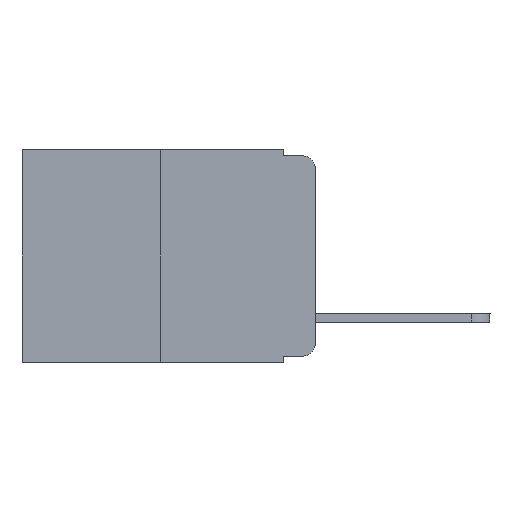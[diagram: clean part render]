
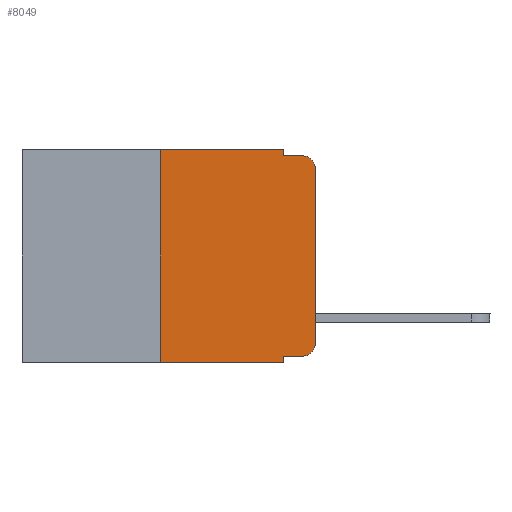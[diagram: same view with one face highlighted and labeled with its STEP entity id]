
A CAD part, left-side view. The second image highlights one B-rep face of the part: STEP entity #8049.
In plain terms, the highlighted planar face has unit normal (-1, 0, 0).
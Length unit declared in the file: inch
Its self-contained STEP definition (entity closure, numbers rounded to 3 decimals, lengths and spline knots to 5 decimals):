
#167 = VECTOR ( 'NONE', #13975, 39.37008 ) ;
#238 = EDGE_CURVE ( 'NONE', #725, #4307, #11123, .T. ) ;
#259 = LINE ( 'NONE', #12932, #1008 ) ;
#273 = LINE ( 'NONE', #460, #11075 ) ;
#423 = VERTEX_POINT ( 'NONE', #4367 ) ;
#460 = CARTESIAN_POINT ( 'NONE',  ( 0., 0.473, 0. ) ) ;
#542 = LINE ( 'NONE', #11695, #167 ) ;
#674 = EDGE_CURVE ( 'NONE', #6164, #3727, #14731, .T. ) ;
#712 = CARTESIAN_POINT ( 'NONE',  ( 0., 0.02, -0.01 ) ) ;
#725 = VERTEX_POINT ( 'NONE', #7876 ) ;
#894 = ORIENTED_EDGE ( 'NONE', *, *, #15032, .T. ) ;
#1008 = VECTOR ( 'NONE', #12884, 39.37008 ) ;
#1167 = DIRECTION ( 'NONE',  ( 0., 0., -1. ) ) ;
#1240 = VECTOR ( 'NONE', #3168, 39.37008 ) ;
#1358 = CARTESIAN_POINT ( 'NONE',  ( 0., 0.473, -0.343 ) ) ;
#1470 = CARTESIAN_POINT ( 'NONE',  ( 0., 0.051, 0. ) ) ;
#1743 = AXIS2_PLACEMENT_3D ( 'NONE', #9696, #6143, #3872 ) ;
#1749 = EDGE_CURVE ( 'NONE', #423, #4333, #7086, .T. ) ;
#1755 = VECTOR ( 'NONE', #3588, 39.37008 ) ;
#1816 = LINE ( 'NONE', #6655, #1240 ) ;
#1818 = VERTEX_POINT ( 'NONE', #5505 ) ;
#1842 = DIRECTION ( 'NONE',  ( 0., -1., 0. ) ) ;
#2102 = FACE_OUTER_BOUND ( 'NONE', #4082, .T. ) ;
#2313 = CARTESIAN_POINT ( 'NONE',  ( 0., 0.02, -0.313 ) ) ;
#2544 = AXIS2_PLACEMENT_3D ( 'NONE', #6392, #9747, #6288 ) ;
#2685 = CARTESIAN_POINT ( 'NONE',  ( 0., 0., -0.313 ) ) ;
#2924 = ORIENTED_EDGE ( 'NONE', *, *, #674, .T. ) ;
#3017 = VERTEX_POINT ( 'NONE', #6673 ) ;
#3168 = DIRECTION ( 'NONE',  ( 0., -1., 0. ) ) ;
#3588 = DIRECTION ( 'NONE',  ( 0., -1., 0. ) ) ;
#3604 = CARTESIAN_POINT ( 'NONE',  ( 0., 0.051, -0.333 ) ) ;
#3661 = CARTESIAN_POINT ( 'NONE',  ( 0., 0.25, 0. ) ) ;
#3727 = VERTEX_POINT ( 'NONE', #14265 ) ;
#3760 = ORIENTED_EDGE ( 'NONE', *, *, #12915, .F. ) ;
#3872 = DIRECTION ( 'NONE',  ( 0., 0., -1. ) ) ;
#4082 = EDGE_LOOP ( 'NONE', ( #894, #4357, #5508, #11124, #3760, #12604, #7837, #5061, #2924, #10847 ) ) ;
#4221 = EDGE_CURVE ( 'NONE', #6164, #1818, #542, .T. ) ;
#4307 = VERTEX_POINT ( 'NONE', #8518 ) ;
#4327 = CIRCLE ( 'NONE', #5740, 0.02 ) ;
#4333 = VERTEX_POINT ( 'NONE', #3661 ) ;
#4337 = VERTEX_POINT ( 'NONE', #2685 ) ;
#4357 = ORIENTED_EDGE ( 'NONE', *, *, #9802, .T. ) ;
#4367 = CARTESIAN_POINT ( 'NONE',  ( 0., 0.25, -0.343 ) ) ;
#4740 = VECTOR ( 'NONE', #1842, 39.37008 ) ;
#5061 = ORIENTED_EDGE ( 'NONE', *, *, #4221, .F. ) ;
#5170 = EDGE_CURVE ( 'NONE', #4307, #13240, #1816, .T. ) ;
#5505 = CARTESIAN_POINT ( 'NONE',  ( 0., 0.051, -0.343 ) ) ;
#5508 = ORIENTED_EDGE ( 'NONE', *, *, #5170, .F. ) ;
#5531 = CIRCLE ( 'NONE', #2544, 0.02 ) ;
#5740 = AXIS2_PLACEMENT_3D ( 'NONE', #2313, #11634, #1167 ) ;
#5993 = VECTOR ( 'NONE', #11097, 39.37008 ) ;
#6143 = DIRECTION ( 'NONE',  ( 1., 0., 0. ) ) ;
#6164 = VERTEX_POINT ( 'NONE', #3604 ) ;
#6265 = CARTESIAN_POINT ( 'NONE',  ( 0., 0.25, 0. ) ) ;
#6288 = DIRECTION ( 'NONE',  ( 0., 0., -1. ) ) ;
#6392 = CARTESIAN_POINT ( 'NONE',  ( 0., 0.02, -0.03 ) ) ;
#6655 = CARTESIAN_POINT ( 'NONE',  ( 0., 0.051, -0.01 ) ) ;
#6673 = CARTESIAN_POINT ( 'NONE',  ( 0., 0., -0.03 ) ) ;
#7086 = LINE ( 'NONE', #6265, #5993 ) ;
#7837 = ORIENTED_EDGE ( 'NONE', *, *, #15109, .T. ) ;
#7876 = CARTESIAN_POINT ( 'NONE',  ( 0., 0.051, 0. ) ) ;
#8049 = ADVANCED_FACE ( 'NONE', ( #2102 ), #13081, .F. ) ;
#8518 = CARTESIAN_POINT ( 'NONE',  ( 0., 0.051, -0.01 ) ) ;
#9696 = CARTESIAN_POINT ( 'NONE',  ( 0., 0.473, 0. ) ) ;
#9747 = DIRECTION ( 'NONE',  ( -1., 0., 0. ) ) ;
#9802 = EDGE_CURVE ( 'NONE', #3017, #13240, #5531, .T. ) ;
#10847 = ORIENTED_EDGE ( 'NONE', *, *, #13525, .T. ) ;
#11075 = VECTOR ( 'NONE', #14485, 39.37008 ) ;
#11097 = DIRECTION ( 'NONE',  ( 0., 0., 1. ) ) ;
#11123 = LINE ( 'NONE', #1470, #12013 ) ;
#11124 = ORIENTED_EDGE ( 'NONE', *, *, #238, .F. ) ;
#11420 = LINE ( 'NONE', #1358, #1755 ) ;
#11634 = DIRECTION ( 'NONE',  ( -1., 0., 0. ) ) ;
#11695 = CARTESIAN_POINT ( 'NONE',  ( 0., 0.051, 0. ) ) ;
#11970 = DIRECTION ( 'NONE',  ( 0., 0., -1. ) ) ;
#12013 = VECTOR ( 'NONE', #11970, 39.37008 ) ;
#12604 = ORIENTED_EDGE ( 'NONE', *, *, #1749, .F. ) ;
#12884 = DIRECTION ( 'NONE',  ( 0., 0., 1. ) ) ;
#12915 = EDGE_CURVE ( 'NONE', #4333, #725, #273, .T. ) ;
#12932 = CARTESIAN_POINT ( 'NONE',  ( 0., 0., 0. ) ) ;
#13081 = PLANE ( 'NONE',  #1743 ) ;
#13240 = VERTEX_POINT ( 'NONE', #712 ) ;
#13525 = EDGE_CURVE ( 'NONE', #3727, #4337, #4327, .T. ) ;
#13975 = DIRECTION ( 'NONE',  ( 0., 0., -1. ) ) ;
#14265 = CARTESIAN_POINT ( 'NONE',  ( 0., 0.02, -0.333 ) ) ;
#14485 = DIRECTION ( 'NONE',  ( 0., -1., 0. ) ) ;
#14607 = CARTESIAN_POINT ( 'NONE',  ( 0., 0.051, -0.333 ) ) ;
#14731 = LINE ( 'NONE', #14607, #4740 ) ;
#15032 = EDGE_CURVE ( 'NONE', #4337, #3017, #259, .T. ) ;
#15109 = EDGE_CURVE ( 'NONE', #423, #1818, #11420, .T. ) ;
